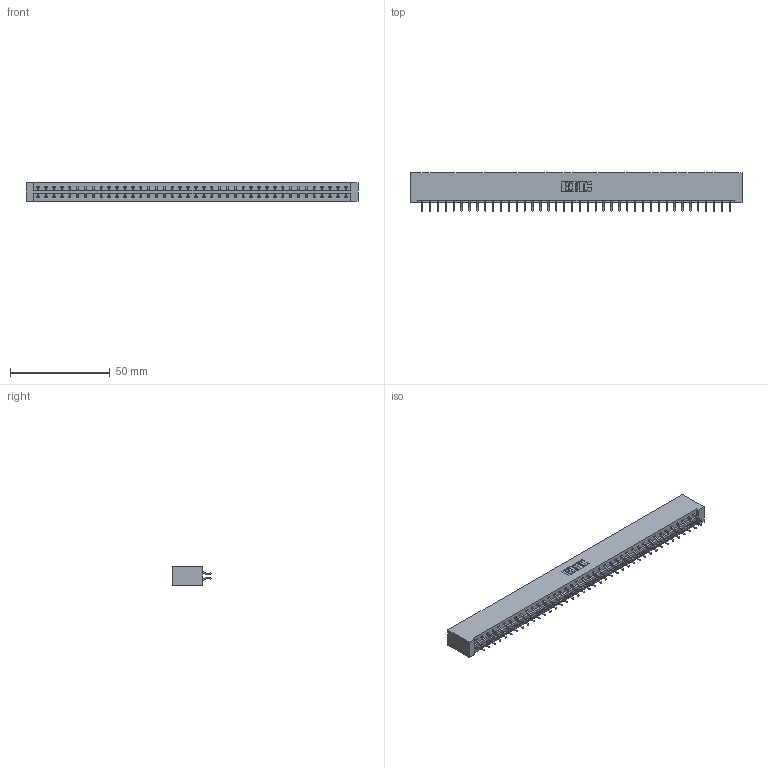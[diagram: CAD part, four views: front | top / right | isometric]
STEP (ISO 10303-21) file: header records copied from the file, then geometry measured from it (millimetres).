
FILE_DESCRIPTION (( 'STEP AP203' ), '1' );
FILE_NAME ('833-080-556-201.STEP', '2020-06-05T22:20:37', ( '' ), ( '' ), 'SwSTEP 2.0', 'SolidWorks 2020', '' );
FILE_SCHEMA (( 'CONFIG_CONTROL_DESIGN' ));
Length unit declared in the file: inch
Products named in the file (3): 833 Part_Lugless; 833-080-556-201; 345-292-001_556 Tail
Assembly tree (81 placements, depth 2):
  833-080-556-201
    833 Part_Lugless
    345-292-001_556 Tail  x80
Bounding box: 166.75 x 19.57 x 9.4 mm (x, y, z)
Volume: 17634.7 mm3; surface area: 20772.5 mm2
Topology: 81 solids, 81 shells, 4746 faces, 14127 edges, 9310 vertices
Faces by surface type: plane 3266, cylinder 1480
Entity records: 25935 total; most frequent: CARTESIAN_POINT 4314, ORIENTED_EDGE 4238, DIRECTION 3671, EDGE_CURVE 2119, VECTOR 1991, LINE 1991, VERTEX_POINT 1410, AXIS2_PLACEMENT_3D 840
